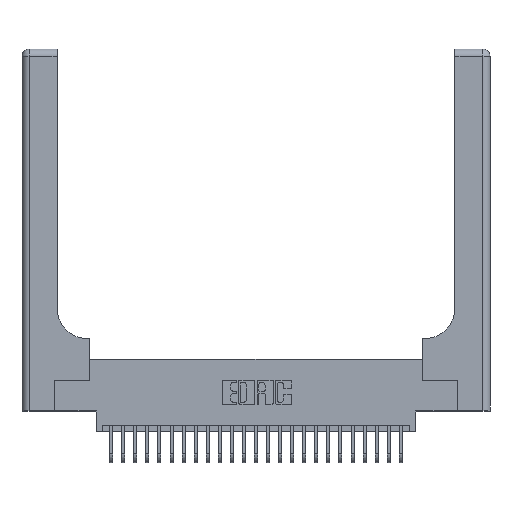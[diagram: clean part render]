
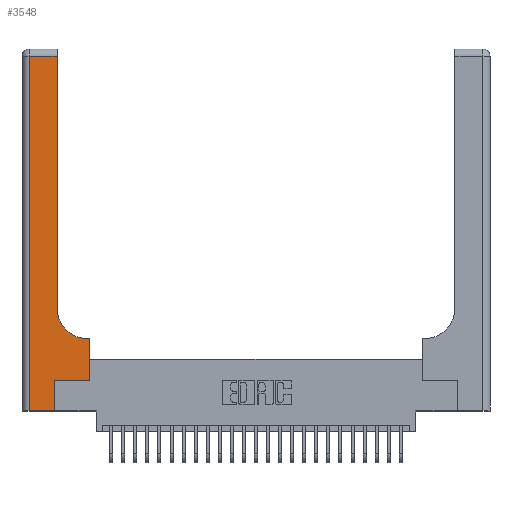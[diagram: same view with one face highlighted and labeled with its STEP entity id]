
A CAD part, top view. The second image highlights one B-rep face of the part: STEP entity #3548.
In plain terms, the highlighted planar face has unit normal (0, 0, 1).
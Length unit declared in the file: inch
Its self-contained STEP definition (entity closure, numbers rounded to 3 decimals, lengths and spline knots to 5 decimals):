
#120 = CARTESIAN_POINT ( 'NONE',  ( 0.2915, 0.6, 0.37 ) ) ;
#324 = VERTEX_POINT ( 'NONE', #6557 ) ;
#383 = LINE ( 'NONE', #14374, #11770 ) ;
#390 = CARTESIAN_POINT ( 'NONE',  ( 0.2915, 3., 0.37 ) ) ;
#513 = VECTOR ( 'NONE', #9172, 39.37008 ) ;
#1056 = CARTESIAN_POINT ( 'NONE',  ( 0.269, 0.25, 0.37 ) ) ;
#1236 = EDGE_CURVE ( 'NONE', #14128, #324, #23679, .T. ) ;
#1410 = VECTOR ( 'NONE', #25695, 39.37008 ) ;
#2247 = ORIENTED_EDGE ( 'NONE', *, *, #26875, .T. ) ;
#2357 = LINE ( 'NONE', #120, #7721 ) ;
#2549 = DIRECTION ( 'NONE',  ( -1., 0., 0. ) ) ;
#3548 = ADVANCED_FACE ( 'NONE', ( #18551 ), #9866, .F. ) ;
#4300 = ORIENTED_EDGE ( 'NONE', *, *, #4734, .T. ) ;
#4689 = EDGE_CURVE ( 'NONE', #17117, #14128, #21635, .T. ) ;
#4734 = EDGE_CURVE ( 'NONE', #24855, #16192, #2357, .T. ) ;
#5404 = DIRECTION ( 'NONE',  ( -1., 0., 0. ) ) ;
#5673 = DIRECTION ( 'NONE',  ( 0., 0., -1. ) ) ;
#5890 = CARTESIAN_POINT ( 'NONE',  ( 0.5585, 0.6, 0.37 ) ) ;
#6173 = VERTEX_POINT ( 'NONE', #14949 ) ;
#6301 = EDGE_CURVE ( 'NONE', #6173, #10389, #9764, .T. ) ;
#6402 = CARTESIAN_POINT ( 'NONE',  ( 0., 2.94, 0.37 ) ) ;
#6557 = CARTESIAN_POINT ( 'NONE',  ( 0.269, 0.25, 0.37 ) ) ;
#7466 = ORIENTED_EDGE ( 'NONE', *, *, #1236, .T. ) ;
#7721 = VECTOR ( 'NONE', #2549, 39.37008 ) ;
#7799 = CARTESIAN_POINT ( 'NONE',  ( 0.2915, 0.85, 0.37 ) ) ;
#8190 = EDGE_CURVE ( 'NONE', #10389, #17117, #383, .T. ) ;
#8213 = CIRCLE ( 'NONE', #12773, 0.25 ) ;
#8523 = ORIENTED_EDGE ( 'NONE', *, *, #27956, .T. ) ;
#8878 = ORIENTED_EDGE ( 'NONE', *, *, #16674, .T. ) ;
#9070 = DIRECTION ( 'NONE',  ( 0., 1., 0. ) ) ;
#9172 = DIRECTION ( 'NONE',  ( 0., 1., 0. ) ) ;
#9186 = LINE ( 'NONE', #390, #26157 ) ;
#9260 = CARTESIAN_POINT ( 'NONE',  ( 0.269, 0., 0.37 ) ) ;
#9764 = LINE ( 'NONE', #6402, #10467 ) ;
#9866 = PLANE ( 'NONE',  #26804 ) ;
#9879 = CARTESIAN_POINT ( 'NONE',  ( 0.06, 0., 0.37 ) ) ;
#10389 = VERTEX_POINT ( 'NONE', #19913 ) ;
#10467 = VECTOR ( 'NONE', #21897, 39.37008 ) ;
#11369 = CARTESIAN_POINT ( 'NONE',  ( 0., 0., 0.37 ) ) ;
#11770 = VECTOR ( 'NONE', #23256, 39.37008 ) ;
#12773 = AXIS2_PLACEMENT_3D ( 'NONE', #19026, #5673, #21286 ) ;
#13067 = VERTEX_POINT ( 'NONE', #23717 ) ;
#13717 = DIRECTION ( 'NONE',  ( 1., 0., 0. ) ) ;
#14128 = VERTEX_POINT ( 'NONE', #26989 ) ;
#14374 = CARTESIAN_POINT ( 'NONE',  ( 0.06, 3., 0.37 ) ) ;
#14949 = CARTESIAN_POINT ( 'NONE',  ( 0.2915, 2.94, 0.37 ) ) ;
#15895 = EDGE_LOOP ( 'NONE', ( #8523, #19597, #28866, #25493, #7466, #28245, #8878, #4300, #2247 ) ) ;
#16192 = VERTEX_POINT ( 'NONE', #18307 ) ;
#16674 = EDGE_CURVE ( 'NONE', #13067, #24855, #28115, .T. ) ;
#17117 = VERTEX_POINT ( 'NONE', #9879 ) ;
#17128 = VECTOR ( 'NONE', #9070, 39.37008 ) ;
#18307 = CARTESIAN_POINT ( 'NONE',  ( 0.5415, 0.6, 0.37 ) ) ;
#18551 = FACE_OUTER_BOUND ( 'NONE', #15895, .T. ) ;
#18777 = DIRECTION ( 'NONE',  ( 0., 0., -1. ) ) ;
#19026 = CARTESIAN_POINT ( 'NONE',  ( 0.5415, 0.85, 0.37 ) ) ;
#19597 = ORIENTED_EDGE ( 'NONE', *, *, #6301, .T. ) ;
#19913 = CARTESIAN_POINT ( 'NONE',  ( 0.06, 2.94, 0.37 ) ) ;
#20024 = LINE ( 'NONE', #1056, #1410 ) ;
#21286 = DIRECTION ( 'NONE',  ( 1., 0., 0. ) ) ;
#21635 = LINE ( 'NONE', #11369, #26085 ) ;
#21897 = DIRECTION ( 'NONE',  ( -1., 0., 0. ) ) ;
#22359 = CARTESIAN_POINT ( 'NONE',  ( 0.5585, 0.25, 0.37 ) ) ;
#23256 = DIRECTION ( 'NONE',  ( 0., -1., 0. ) ) ;
#23679 = LINE ( 'NONE', #9260, #513 ) ;
#23717 = CARTESIAN_POINT ( 'NONE',  ( 0.5585, 0.25, 0.37 ) ) ;
#24855 = VERTEX_POINT ( 'NONE', #5890 ) ;
#25346 = CARTESIAN_POINT ( 'NONE',  ( 0., 3., 0.37 ) ) ;
#25493 = ORIENTED_EDGE ( 'NONE', *, *, #4689, .T. ) ;
#25695 = DIRECTION ( 'NONE',  ( 1., 0., 0. ) ) ;
#26085 = VECTOR ( 'NONE', #13717, 39.37008 ) ;
#26157 = VECTOR ( 'NONE', #27252, 39.37008 ) ;
#26804 = AXIS2_PLACEMENT_3D ( 'NONE', #25346, #18777, #5404 ) ;
#26875 = EDGE_CURVE ( 'NONE', #16192, #28622, #8213, .T. ) ;
#26893 = EDGE_CURVE ( 'NONE', #324, #13067, #20024, .T. ) ;
#26989 = CARTESIAN_POINT ( 'NONE',  ( 0.269, 0., 0.37 ) ) ;
#27252 = DIRECTION ( 'NONE',  ( 0., 1., 0. ) ) ;
#27956 = EDGE_CURVE ( 'NONE', #28622, #6173, #9186, .T. ) ;
#28115 = LINE ( 'NONE', #22359, #17128 ) ;
#28245 = ORIENTED_EDGE ( 'NONE', *, *, #26893, .T. ) ;
#28622 = VERTEX_POINT ( 'NONE', #7799 ) ;
#28866 = ORIENTED_EDGE ( 'NONE', *, *, #8190, .T. ) ;
